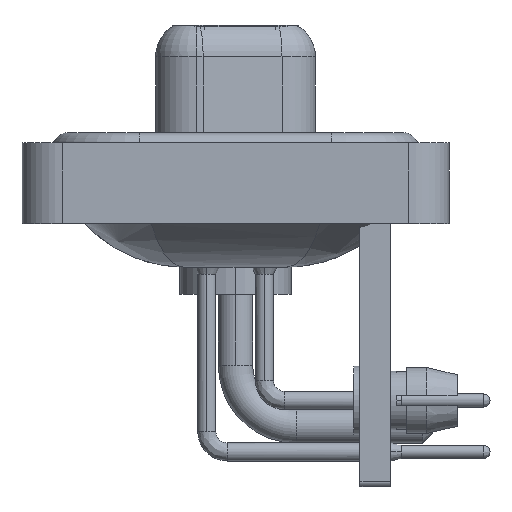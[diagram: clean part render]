
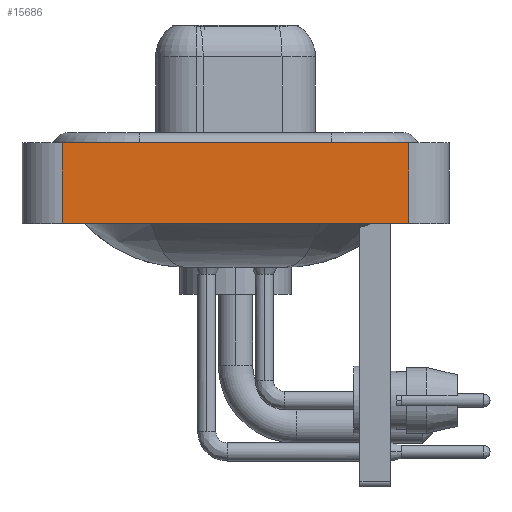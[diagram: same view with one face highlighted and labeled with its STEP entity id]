
A CAD part, left-side view. The second image highlights one B-rep face of the part: STEP entity #15686.
In plain terms, the highlighted planar face has unit normal (-1, 0, 0).
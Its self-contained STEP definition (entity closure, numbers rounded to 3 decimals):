
#206 = LINE ( 'NONE', #19387, #14930 ) ;
#504 = ORIENTED_EDGE ( 'NONE', *, *, #1410, .T. ) ;
#1101 = CARTESIAN_POINT ( 'NONE',  ( -7.3, -8.55, -3.6 ) ) ;
#1410 = EDGE_CURVE ( 'NONE', #7676, #12702, #17880, .T. ) ;
#2219 = DIRECTION ( 'NONE',  ( 0., -1., 0. ) ) ;
#2590 = DIRECTION ( 'NONE',  ( 0., -1., 0. ) ) ;
#3163 = CARTESIAN_POINT ( 'NONE',  ( -7.3, -8.55, -3.6 ) ) ;
#3372 = DIRECTION ( 'NONE',  ( 0., 0., 1. ) ) ;
#6724 = CARTESIAN_POINT ( 'NONE',  ( -7.3, 8.55, -3.6 ) ) ;
#7676 = VERTEX_POINT ( 'NONE', #16744 ) ;
#8557 = VECTOR ( 'NONE', #2590, 1000. ) ;
#10160 = VECTOR ( 'NONE', #18259, 1000. ) ;
#10204 = DIRECTION ( 'NONE',  ( -1., 0., 0. ) ) ;
#10625 = ORIENTED_EDGE ( 'NONE', *, *, #17637, .T. ) ;
#11099 = ORIENTED_EDGE ( 'NONE', *, *, #15391, .F. ) ;
#11766 = AXIS2_PLACEMENT_3D ( 'NONE', #11948, #10204, #15828 ) ;
#11948 = CARTESIAN_POINT ( 'NONE',  ( -7.3, -8.55, -3.6 ) ) ;
#12001 = ORIENTED_EDGE ( 'NONE', *, *, #15304, .F. ) ;
#12702 = VERTEX_POINT ( 'NONE', #3163 ) ;
#13585 = FACE_OUTER_BOUND ( 'NONE', #13867, .T. ) ;
#13860 = CARTESIAN_POINT ( 'NONE',  ( -7.3, 8.55, 0.4 ) ) ;
#13867 = EDGE_LOOP ( 'NONE', ( #10625, #12001, #11099, #504 ) ) ;
#14625 = VERTEX_POINT ( 'NONE', #23058 ) ;
#14631 = LINE ( 'NONE', #1101, #17112 ) ;
#14930 = VECTOR ( 'NONE', #2219, 1000. ) ;
#15304 = EDGE_CURVE ( 'NONE', #16620, #14625, #206, .T. ) ;
#15391 = EDGE_CURVE ( 'NONE', #7676, #16620, #16103, .T. ) ;
#15686 = ADVANCED_FACE ( 'NONE', ( #13585 ), #19592, .T. ) ;
#15828 = DIRECTION ( 'NONE',  ( 0., 0., 1. ) ) ;
#16103 = LINE ( 'NONE', #6724, #10160 ) ;
#16620 = VERTEX_POINT ( 'NONE', #13860 ) ;
#16744 = CARTESIAN_POINT ( 'NONE',  ( -7.3, 8.55, -3.6 ) ) ;
#17112 = VECTOR ( 'NONE', #3372, 1000. ) ;
#17637 = EDGE_CURVE ( 'NONE', #12702, #14625, #14631, .T. ) ;
#17880 = LINE ( 'NONE', #23638, #8557 ) ;
#18259 = DIRECTION ( 'NONE',  ( 0., 0., 1. ) ) ;
#19387 = CARTESIAN_POINT ( 'NONE',  ( -7.3, -8.55, 0.4 ) ) ;
#19592 = PLANE ( 'NONE',  #11766 ) ;
#23058 = CARTESIAN_POINT ( 'NONE',  ( -7.3, -8.55, 0.4 ) ) ;
#23638 = CARTESIAN_POINT ( 'NONE',  ( -7.3, -8.55, -3.6 ) ) ;
